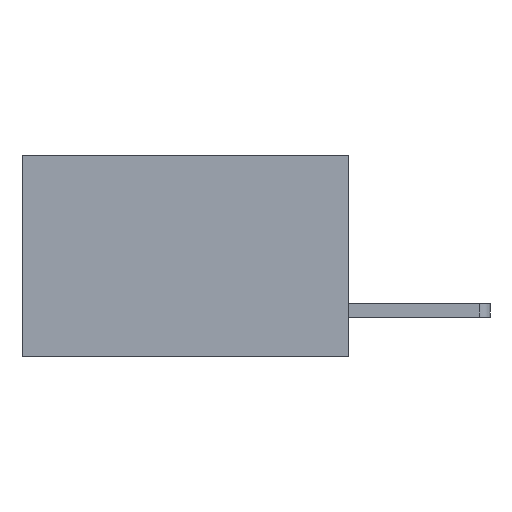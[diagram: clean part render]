
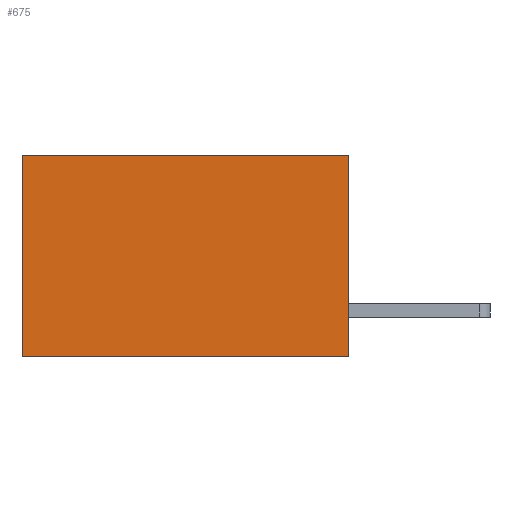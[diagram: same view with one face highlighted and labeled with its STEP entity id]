
A CAD part, left-side view. The second image highlights one B-rep face of the part: STEP entity #675.
In plain terms, the highlighted planar face has unit normal (-1, 0, 0).
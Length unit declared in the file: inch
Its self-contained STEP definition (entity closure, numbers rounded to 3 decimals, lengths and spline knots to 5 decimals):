
#105 = ORIENTED_EDGE ( 'NONE', *, *, #7869, .T. ) ;
#127 = VERTEX_POINT ( 'NONE', #6072 ) ;
#285 = LINE ( 'NONE', #7552, #7788 ) ;
#360 = ORIENTED_EDGE ( 'NONE', *, *, #2733, .F. ) ;
#471 = LINE ( 'NONE', #728, #3852 ) ;
#477 = ORIENTED_EDGE ( 'NONE', *, *, #7386, .F. ) ;
#564 = ORIENTED_EDGE ( 'NONE', *, *, #9166, .T. ) ;
#675 = ADVANCED_FACE ( 'NONE', ( #9267 ), #5214, .F. ) ;
#686 = DIRECTION ( 'NONE',  ( 1., 0., 0. ) ) ;
#728 = CARTESIAN_POINT ( 'NONE',  ( 0.2615, 0., 0. ) ) ;
#924 = CARTESIAN_POINT ( 'NONE',  ( 0.2615, 0.6, -0.37 ) ) ;
#1283 = CARTESIAN_POINT ( 'NONE',  ( 0.2615, 0., 0. ) ) ;
#1305 = CARTESIAN_POINT ( 'NONE',  ( 0.2615, 0., -0.37 ) ) ;
#1762 = LINE ( 'NONE', #5829, #9162 ) ;
#2404 = CARTESIAN_POINT ( 'NONE',  ( 0.2615, 0., -0.37 ) ) ;
#2448 = VERTEX_POINT ( 'NONE', #924 ) ;
#2733 = EDGE_CURVE ( 'NONE', #4430, #2448, #285, .T. ) ;
#3307 = CARTESIAN_POINT ( 'NONE',  ( 0.2615, 0., -0.37 ) ) ;
#3704 = DIRECTION ( 'NONE',  ( 0., 1., 0. ) ) ;
#3775 = EDGE_LOOP ( 'NONE', ( #105, #360, #477, #564 ) ) ;
#3852 = VECTOR ( 'NONE', #5315, 39.37008 ) ;
#3968 = VECTOR ( 'NONE', #6558, 39.37008 ) ;
#4430 = VERTEX_POINT ( 'NONE', #3307 ) ;
#4577 = VERTEX_POINT ( 'NONE', #1283 ) ;
#5214 = PLANE ( 'NONE',  #8772 ) ;
#5315 = DIRECTION ( 'NONE',  ( 0., 1., 0. ) ) ;
#5829 = CARTESIAN_POINT ( 'NONE',  ( 0.2615, 0.6, -0.37 ) ) ;
#5858 = DIRECTION ( 'NONE',  ( 0., 0., -1. ) ) ;
#6072 = CARTESIAN_POINT ( 'NONE',  ( 0.2615, 0.6, 0. ) ) ;
#6558 = DIRECTION ( 'NONE',  ( 0., 0., -1. ) ) ;
#7386 = EDGE_CURVE ( 'NONE', #4577, #4430, #9128, .T. ) ;
#7552 = CARTESIAN_POINT ( 'NONE',  ( 0.2615, 0., -0.37 ) ) ;
#7788 = VECTOR ( 'NONE', #3704, 39.37008 ) ;
#7869 = EDGE_CURVE ( 'NONE', #127, #2448, #1762, .T. ) ;
#8691 = DIRECTION ( 'NONE',  ( 0., 0., -1. ) ) ;
#8772 = AXIS2_PLACEMENT_3D ( 'NONE', #2404, #686, #8691 ) ;
#9128 = LINE ( 'NONE', #1305, #3968 ) ;
#9162 = VECTOR ( 'NONE', #5858, 39.37008 ) ;
#9166 = EDGE_CURVE ( 'NONE', #4577, #127, #471, .T. ) ;
#9267 = FACE_OUTER_BOUND ( 'NONE', #3775, .T. ) ;
